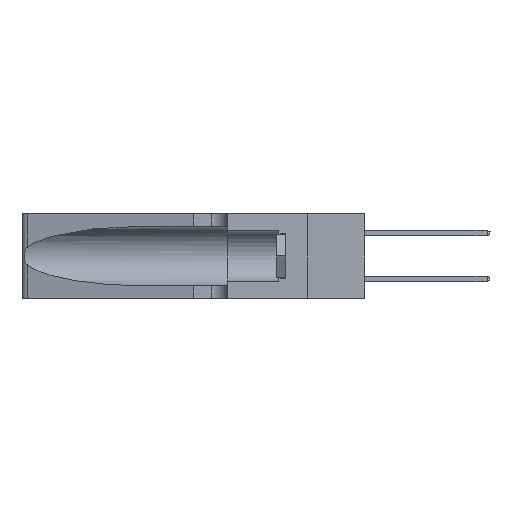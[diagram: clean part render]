
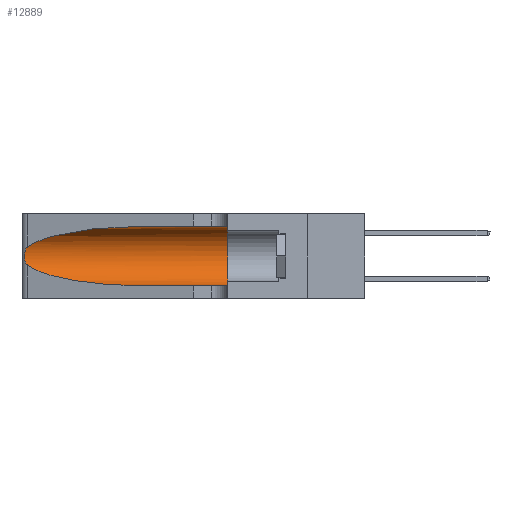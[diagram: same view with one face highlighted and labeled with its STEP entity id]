
A CAD part, left-side view. The second image highlights one B-rep face of the part: STEP entity #12889.
In plain terms, the highlighted cylindrical face has radius 3.308 mm (diameter 6.617 mm), a partial arc.
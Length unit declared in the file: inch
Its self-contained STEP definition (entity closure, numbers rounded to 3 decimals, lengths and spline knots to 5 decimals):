
#210 = CARTESIAN_POINT ( 'NONE',  ( 0.26075, 1.23896, 0.19203 ) ) ;
#611 = CARTESIAN_POINT ( 'NONE',  ( 0.18966, 0.96281, 0.05475 ) ) ;
#1394 = DIRECTION ( 'NONE',  ( 0., -1., 0. ) ) ;
#3561 = CARTESIAN_POINT ( 'NONE',  ( 0.25639, 1.23184, 0.21858 ) ) ;
#4058 = EDGE_CURVE ( 'NONE', #20386, #38115, #10088, .T. ) ;
#5038 = AXIS2_PLACEMENT_3D ( 'NONE', #18297, #35564, #7846 ) ;
#6628 = CARTESIAN_POINT ( 'NONE',  ( 0.1305, 1.61858, 0.31525 ) ) ;
#6631 = CARTESIAN_POINT ( 'NONE',  ( 0.25555, 1.22994, 0.2215 ) ) ;
#7067 = CARTESIAN_POINT ( 'NONE',  ( 0.26018, 1.23835, 0.19895 ) ) ;
#7221 = CARTESIAN_POINT ( 'NONE',  ( 0.25487, 1.22718, 0.22369 ) ) ;
#7585 = CARTESIAN_POINT ( 'NONE',  ( 0.25487, 1.22718, 0.14631 ) ) ;
#7846 = DIRECTION ( 'NONE',  ( 0., 0., 1. ) ) ;
#9131 = ORIENTED_EDGE ( 'NONE', *, *, #31336, .T. ) ;
#10088 = CIRCLE ( 'NONE', #5038, 0.13025 ) ;
#10531 = CARTESIAN_POINT ( 'NONE',  ( 0.26017, 1.23833, 0.17102 ) ) ;
#10896 = CYLINDRICAL_SURFACE ( 'NONE', #43032, 0.13025 ) ;
#10906 =( BOUNDED_CURVE ( )  B_SPLINE_CURVE ( 3, ( #35669, #11576, #611, #21262 ),
 .UNSPECIFIED., .F., .F. ) 
 B_SPLINE_CURVE_WITH_KNOTS ( ( 4, 4 ),
 ( 3.44316, 4.71239 ),
 .UNSPECIFIED. ) 
 CURVE ( )  GEOMETRIC_REPRESENTATION_ITEM ( )  RATIONAL_B_SPLINE_CURVE ( ( 1., 0.87, 0.87, 1. ) ) 
 REPRESENTATION_ITEM ( '' )  );
#11576 = CARTESIAN_POINT ( 'NONE',  ( 0.2373, 1.15595, 0.08982 ) ) ;
#11638 = ORIENTED_EDGE ( 'NONE', *, *, #32475, .T. ) ;
#12889 = ADVANCED_FACE ( 'NONE', ( #31513 ), #10896, .F. ) ;
#12899 = CARTESIAN_POINT ( 'NONE',  ( 0.25487, 1.22718, 0.22369 ) ) ;
#13847 = CARTESIAN_POINT ( 'NONE',  ( 0.25487, 1.22718, 0.22369 ) ) ;
#14663 = VERTEX_POINT ( 'NONE', #40267 ) ;
#14667 = ORIENTED_EDGE ( 'NONE', *, *, #4058, .F. ) ;
#14734 = CARTESIAN_POINT ( 'NONE',  ( 0.25789, 1.23486, 0.15765 ) ) ;
#16098 = CARTESIAN_POINT ( 'NONE',  ( 0.18966, 0.96281, 0.31525 ) ) ;
#17542 = ORIENTED_EDGE ( 'NONE', *, *, #27182, .F. ) ;
#17603 = ORIENTED_EDGE ( 'NONE', *, *, #35928, .T. ) ;
#18264 = EDGE_LOOP ( 'NONE', ( #17603, #24298, #9131, #11638, #14667, #17542 ) ) ;
#18297 = CARTESIAN_POINT ( 'NONE',  ( 0.1305, 0.35, 0.185 ) ) ;
#18417 = CARTESIAN_POINT ( 'NONE',  ( 0.1305, 0.35, 0.31525 ) ) ;
#19047 = VECTOR ( 'NONE', #39487, 39.37008 ) ;
#20386 = VERTEX_POINT ( 'NONE', #18417 ) ;
#21262 = CARTESIAN_POINT ( 'NONE',  ( 0.1305, 0.72297, 0.05475 ) ) ;
#21711 = CARTESIAN_POINT ( 'NONE',  ( 0.25639, 1.23186, 0.15144 ) ) ;
#23036 = CARTESIAN_POINT ( 'NONE',  ( 0.2373, 1.15595, 0.28018 ) ) ;
#24298 = ORIENTED_EDGE ( 'NONE', *, *, #35016, .T. ) ;
#24580 = DIRECTION ( 'NONE',  ( 0., -1., 0. ) ) ;
#25125 = LINE ( 'NONE', #41735, #39243 ) ;
#25875 = DIRECTION ( 'NONE',  ( 0., 0., -1. ) ) ;
#26048 = VERTEX_POINT ( 'NONE', #7221 ) ;
#27047 = B_SPLINE_CURVE_WITH_KNOTS ( 'NONE', 3,
 ( #13847, #6631, #3561, #27809, #38422, #7067, #210, #44810, #10531, #37823, #14734, #21711, #38882, #35668 ),
 .UNSPECIFIED., .F., .F.,
 ( 4, 2, 2, 2, 2, 2, 4 ),
 ( 0., 0.00027, 0.00053, 0.00107, 0.0016, 0.00187, 0.00214 ),
 .UNSPECIFIED. ) ;
#27182 = EDGE_CURVE ( 'NONE', #38011, #20386, #39110, .T. ) ;
#27598 = CARTESIAN_POINT ( 'NONE',  ( 0.1305, 0.72297, 0.31525 ) ) ;
#27809 = CARTESIAN_POINT ( 'NONE',  ( 0.25787, 1.23484, 0.2124 ) ) ;
#28053 = CARTESIAN_POINT ( 'NONE',  ( 0.1305, 0.35, 0.05475 ) ) ;
#31336 = EDGE_CURVE ( 'NONE', #43797, #14663, #10906, .T. ) ;
#31513 = FACE_OUTER_BOUND ( 'NONE', #18264, .T. ) ;
#32475 = EDGE_CURVE ( 'NONE', #14663, #38115, #25125, .T. ) ;
#35016 = EDGE_CURVE ( 'NONE', #26048, #43797, #27047, .T. ) ;
#35564 = DIRECTION ( 'NONE',  ( 0., 1., 0. ) ) ;
#35668 = CARTESIAN_POINT ( 'NONE',  ( 0.25487, 1.22718, 0.14631 ) ) ;
#35669 = CARTESIAN_POINT ( 'NONE',  ( 0.25487, 1.22718, 0.14631 ) ) ;
#35928 = EDGE_CURVE ( 'NONE', #38011, #26048, #39848, .T. ) ;
#37823 = CARTESIAN_POINT ( 'NONE',  ( 0.25856, 1.23593, 0.16098 ) ) ;
#38011 = VERTEX_POINT ( 'NONE', #27598 ) ;
#38115 = VERTEX_POINT ( 'NONE', #28053 ) ;
#38422 = CARTESIAN_POINT ( 'NONE',  ( 0.25854, 1.2359, 0.20912 ) ) ;
#38882 = CARTESIAN_POINT ( 'NONE',  ( 0.25555, 1.22993, 0.14849 ) ) ;
#39110 = LINE ( 'NONE', #6628, #19047 ) ;
#39243 = VECTOR ( 'NONE', #24580, 39.37008 ) ;
#39487 = DIRECTION ( 'NONE',  ( 0., -1., 0. ) ) ;
#39848 =( BOUNDED_CURVE ( )  B_SPLINE_CURVE ( 3, ( #44011, #16098, #23036, #12899 ),
 .UNSPECIFIED., .F., .T. ) 
 B_SPLINE_CURVE_WITH_KNOTS ( ( 4, 4 ),
 ( 1.5708, 2.84003 ),
 .UNSPECIFIED. ) 
 CURVE ( )  GEOMETRIC_REPRESENTATION_ITEM ( )  RATIONAL_B_SPLINE_CURVE ( ( 1., 0.87, 0.87, 1. ) ) 
 REPRESENTATION_ITEM ( '' )  );
#40267 = CARTESIAN_POINT ( 'NONE',  ( 0.1305, 0.72297, 0.05475 ) ) ;
#41735 = CARTESIAN_POINT ( 'NONE',  ( 0.1305, 1.61858, 0.05475 ) ) ;
#42880 = CARTESIAN_POINT ( 'NONE',  ( 0.1305, 1.61858, 0.185 ) ) ;
#43032 = AXIS2_PLACEMENT_3D ( 'NONE', #42880, #1394, #25875 ) ;
#43797 = VERTEX_POINT ( 'NONE', #7585 ) ;
#44011 = CARTESIAN_POINT ( 'NONE',  ( 0.1305, 0.72297, 0.31525 ) ) ;
#44810 = CARTESIAN_POINT ( 'NONE',  ( 0.26075, 1.23896, 0.178 ) ) ;
